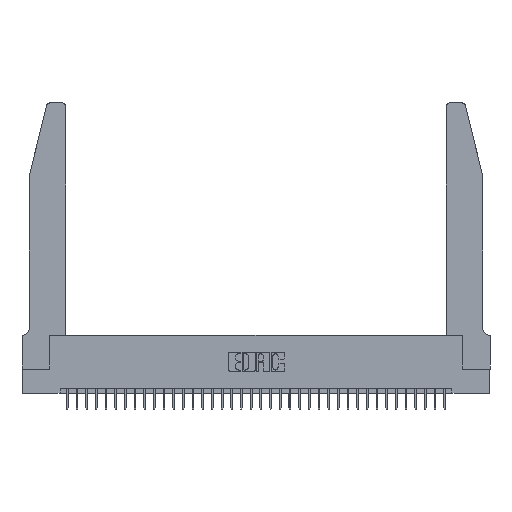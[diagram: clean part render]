
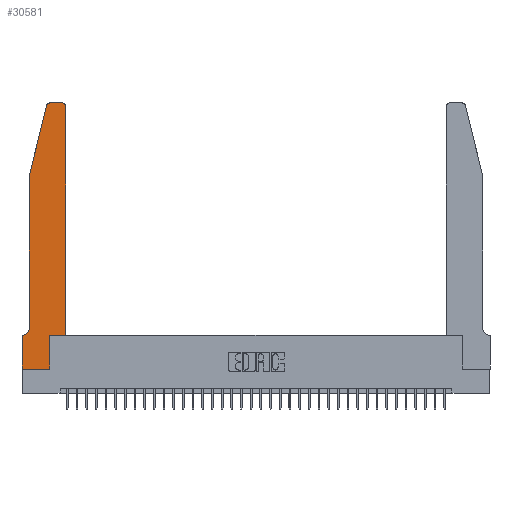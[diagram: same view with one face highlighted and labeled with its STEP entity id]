
A CAD part, top view. The second image highlights one B-rep face of the part: STEP entity #30581.
In plain terms, the highlighted planar face has unit normal (0, 0, 1).
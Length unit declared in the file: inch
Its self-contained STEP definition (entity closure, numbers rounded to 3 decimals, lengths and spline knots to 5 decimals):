
#661 = ORIENTED_EDGE ( 'NONE', *, *, #10173, .T. ) ;
#838 = VERTEX_POINT ( 'NONE', #29168 ) ;
#1311 = CARTESIAN_POINT ( 'NONE',  ( 0.0055, 0.42, 0.37 ) ) ;
#1476 = DIRECTION ( 'NONE',  ( 1., 0., 0. ) ) ;
#1973 = VECTOR ( 'NONE', #16014, 39.37008 ) ;
#2451 = DIRECTION ( 'NONE',  ( -1., 0., 0. ) ) ;
#2546 = ORIENTED_EDGE ( 'NONE', *, *, #31534, .T. ) ;
#2979 = DIRECTION ( 'NONE',  ( 0., -1., 0. ) ) ;
#3107 = CARTESIAN_POINT ( 'NONE',  ( 0.25487, 2.72718, 0.37 ) ) ;
#3557 = CARTESIAN_POINT ( 'NONE',  ( 0.4505, 2.72, 0.37 ) ) ;
#4186 = DIRECTION ( 'NONE',  ( -1., 0., 0. ) ) ;
#4461 = VERTEX_POINT ( 'NONE', #3107 ) ;
#5018 = ORIENTED_EDGE ( 'NONE', *, *, #19158, .T. ) ;
#5292 = LINE ( 'NONE', #10933, #33498 ) ;
#5720 = CARTESIAN_POINT ( 'NONE',  ( 0.4205, 2.72, 0.37 ) ) ;
#6043 = CARTESIAN_POINT ( 'NONE',  ( 0.0755, 2., 0.37 ) ) ;
#6059 = DIRECTION ( 'NONE',  ( 0., 0., 1. ) ) ;
#7420 = CARTESIAN_POINT ( 'NONE',  ( 0., 0., 0.37 ) ) ;
#7902 = CARTESIAN_POINT ( 'NONE',  ( 0., 0., 0.37 ) ) ;
#8295 = CARTESIAN_POINT ( 'NONE',  ( 0.4505, 0.35, 0.37 ) ) ;
#8301 = CARTESIAN_POINT ( 'NONE',  ( 0.4505, 0.35, 0.37 ) ) ;
#8584 = DIRECTION ( 'NONE',  ( 1., 0., 0. ) ) ;
#8968 = ORIENTED_EDGE ( 'NONE', *, *, #23563, .T. ) ;
#9623 = CARTESIAN_POINT ( 'NONE',  ( 0.2865, 0.35, 0.37 ) ) ;
#9954 = EDGE_CURVE ( 'NONE', #36134, #17987, #20007, .T. ) ;
#10001 = LINE ( 'NONE', #6043, #10889 ) ;
#10008 = VECTOR ( 'NONE', #2979, 39.37008 ) ;
#10173 = EDGE_CURVE ( 'NONE', #31910, #4461, #35182, .T. ) ;
#10889 = VECTOR ( 'NONE', #28567, 39.37008 ) ;
#10933 = CARTESIAN_POINT ( 'NONE',  ( 0.0755, 0.35, 0.37 ) ) ;
#11104 = FACE_OUTER_BOUND ( 'NONE', #12283, .T. ) ;
#11148 = DIRECTION ( 'NONE',  ( 0., 1., 0. ) ) ;
#11441 = LINE ( 'NONE', #25442, #25651 ) ;
#11768 = VERTEX_POINT ( 'NONE', #19025 ) ;
#12283 = EDGE_LOOP ( 'NONE', ( #29575, #661, #27999, #33107, #8968, #35668, #25180, #22612, #26837, #2546, #5018, #34816 ) ) ;
#13719 = CIRCLE ( 'NONE', #35340, 0.07 ) ;
#13777 = VERTEX_POINT ( 'NONE', #21511 ) ;
#14106 = EDGE_CURVE ( 'NONE', #28758, #838, #15698, .T. ) ;
#15510 = CARTESIAN_POINT ( 'NONE',  ( 0.0755, 2., 0.37 ) ) ;
#15686 = VERTEX_POINT ( 'NONE', #7902 ) ;
#15698 = CIRCLE ( 'NONE', #24592, 0.03 ) ;
#15796 = VECTOR ( 'NONE', #33122, 39.37008 ) ;
#16014 = DIRECTION ( 'NONE',  ( 1., 0., 0. ) ) ;
#16903 = DIRECTION ( 'NONE',  ( 1., 0., 0. ) ) ;
#17987 = VERTEX_POINT ( 'NONE', #9623 ) ;
#18588 = DIRECTION ( 'NONE',  ( 0., 0., 1. ) ) ;
#19025 = CARTESIAN_POINT ( 'NONE',  ( 0.4505, 0.35, 0.37 ) ) ;
#19074 = EDGE_CURVE ( 'NONE', #15686, #36134, #32015, .T. ) ;
#19158 = EDGE_CURVE ( 'NONE', #11768, #28758, #21133, .T. ) ;
#19295 = EDGE_CURVE ( 'NONE', #4461, #19556, #10001, .T. ) ;
#19411 = CARTESIAN_POINT ( 'NONE',  ( 0.2865, 0.35, 0.37 ) ) ;
#19523 = CARTESIAN_POINT ( 'NONE',  ( 0.2865, 0., 0.37 ) ) ;
#19556 = VERTEX_POINT ( 'NONE', #15510 ) ;
#19982 = EDGE_CURVE ( 'NONE', #13777, #15686, #31574, .T. ) ;
#20007 = LINE ( 'NONE', #19411, #34783 ) ;
#20080 = CARTESIAN_POINT ( 'NONE',  ( 0., 0., 0.37 ) ) ;
#20915 = CARTESIAN_POINT ( 'NONE',  ( 0.0055, 0.35, 0.37 ) ) ;
#21133 = LINE ( 'NONE', #8301, #35035 ) ;
#21230 = DIRECTION ( 'NONE',  ( 0., 0., -1. ) ) ;
#21313 = CARTESIAN_POINT ( 'NONE',  ( 0.284, 2.75, 0.37 ) ) ;
#21511 = CARTESIAN_POINT ( 'NONE',  ( 0., 0.35, 0.37 ) ) ;
#21964 = VECTOR ( 'NONE', #16903, 39.37008 ) ;
#22241 = DIRECTION ( 'NONE',  ( 0., 1., 0. ) ) ;
#22612 = ORIENTED_EDGE ( 'NONE', *, *, #19074, .T. ) ;
#22859 = LINE ( 'NONE', #8295, #21964 ) ;
#23092 = CARTESIAN_POINT ( 'NONE',  ( 0.284, 2.72, 0.37 ) ) ;
#23159 = EDGE_CURVE ( 'NONE', #30490, #13777, #5292, .T. ) ;
#23563 = EDGE_CURVE ( 'NONE', #28030, #30490, #13719, .T. ) ;
#24222 = LINE ( 'NONE', #27599, #15796 ) ;
#24357 = EDGE_CURVE ( 'NONE', #19556, #28030, #11441, .T. ) ;
#24592 = AXIS2_PLACEMENT_3D ( 'NONE', #5720, #25582, #8584 ) ;
#25180 = ORIENTED_EDGE ( 'NONE', *, *, #19982, .T. ) ;
#25442 = CARTESIAN_POINT ( 'NONE',  ( 0.0755, 2., 0.37 ) ) ;
#25582 = DIRECTION ( 'NONE',  ( 0., 0., 1. ) ) ;
#25651 = VECTOR ( 'NONE', #28230, 39.37008 ) ;
#25915 = DIRECTION ( 'NONE',  ( 1., 0., 0. ) ) ;
#26837 = ORIENTED_EDGE ( 'NONE', *, *, #9954, .T. ) ;
#26950 = PLANE ( 'NONE',  #30665 ) ;
#27226 = EDGE_CURVE ( 'NONE', #838, #31910, #24222, .T. ) ;
#27599 = CARTESIAN_POINT ( 'NONE',  ( 0.2605, 2.75, 0.37 ) ) ;
#27999 = ORIENTED_EDGE ( 'NONE', *, *, #19295, .T. ) ;
#28030 = VERTEX_POINT ( 'NONE', #28401 ) ;
#28230 = DIRECTION ( 'NONE',  ( 0., -1., 0. ) ) ;
#28401 = CARTESIAN_POINT ( 'NONE',  ( 0.0755, 0.42, 0.37 ) ) ;
#28567 = DIRECTION ( 'NONE',  ( -0.239, -0.971, 0. ) ) ;
#28758 = VERTEX_POINT ( 'NONE', #3557 ) ;
#29168 = CARTESIAN_POINT ( 'NONE',  ( 0.4205, 2.75, 0.37 ) ) ;
#29575 = ORIENTED_EDGE ( 'NONE', *, *, #27226, .T. ) ;
#30490 = VERTEX_POINT ( 'NONE', #20915 ) ;
#30581 = ADVANCED_FACE ( 'NONE', ( #11104 ), #26950, .T. ) ;
#30665 = AXIS2_PLACEMENT_3D ( 'NONE', #35228, #18588, #1476 ) ;
#31534 = EDGE_CURVE ( 'NONE', #17987, #11768, #22859, .T. ) ;
#31574 = LINE ( 'NONE', #20080, #10008 ) ;
#31910 = VERTEX_POINT ( 'NONE', #21313 ) ;
#32015 = LINE ( 'NONE', #7420, #1973 ) ;
#33107 = ORIENTED_EDGE ( 'NONE', *, *, #24357, .T. ) ;
#33122 = DIRECTION ( 'NONE',  ( -1., 0., 0. ) ) ;
#33498 = VECTOR ( 'NONE', #2451, 39.37008 ) ;
#34783 = VECTOR ( 'NONE', #22241, 39.37008 ) ;
#34816 = ORIENTED_EDGE ( 'NONE', *, *, #14106, .T. ) ;
#35035 = VECTOR ( 'NONE', #11148, 39.37008 ) ;
#35182 = CIRCLE ( 'NONE', #35850, 0.03 ) ;
#35228 = CARTESIAN_POINT ( 'NONE',  ( 0., 0.35, 0.37 ) ) ;
#35340 = AXIS2_PLACEMENT_3D ( 'NONE', #1311, #21230, #4186 ) ;
#35668 = ORIENTED_EDGE ( 'NONE', *, *, #23159, .T. ) ;
#35850 = AXIS2_PLACEMENT_3D ( 'NONE', #23092, #6059, #25915 ) ;
#36134 = VERTEX_POINT ( 'NONE', #19523 ) ;
